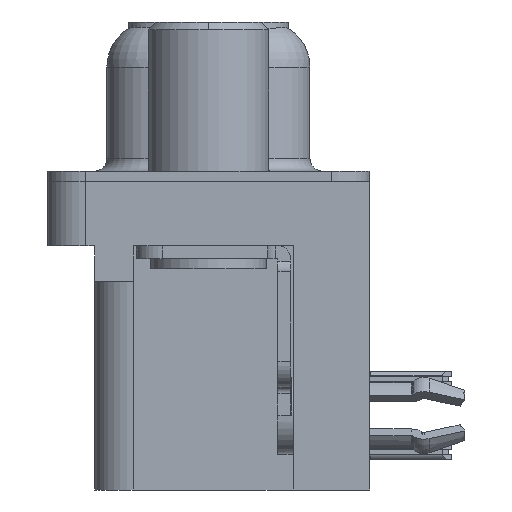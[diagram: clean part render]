
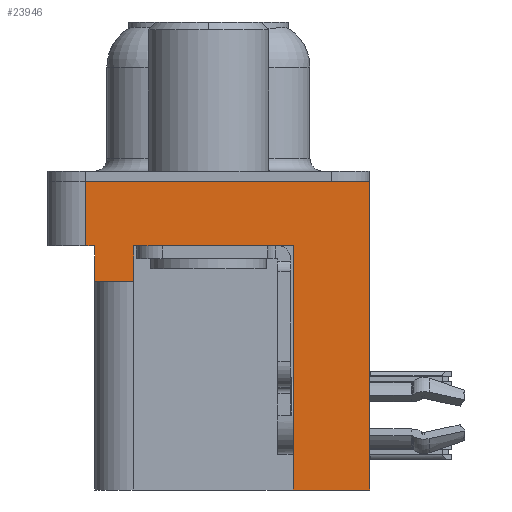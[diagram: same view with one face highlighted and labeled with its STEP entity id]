
A CAD part, left-side view. The second image highlights one B-rep face of the part: STEP entity #23946.
In plain terms, the highlighted planar face has unit normal (-1, 0, 0).
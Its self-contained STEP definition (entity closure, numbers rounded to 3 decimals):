
#235 = EDGE_CURVE ( 'NONE', #28378, #30935, #10967, .T. ) ;
#329 = LINE ( 'NONE', #23512, #26860 ) ;
#631 = AXIS2_PLACEMENT_3D ( 'NONE', #4601, #31173, #10521 ) ;
#839 = CARTESIAN_POINT ( 'NONE',  ( -2.91, 4.425, -3.9 ) ) ;
#1106 = DIRECTION ( 'NONE',  ( 0., 0., 1. ) ) ;
#1242 = LINE ( 'NONE', #29125, #35146 ) ;
#2614 = EDGE_CURVE ( 'NONE', #37680, #4108, #28813, .T. ) ;
#2791 = DIRECTION ( 'NONE',  ( 0., 1., 0. ) ) ;
#3628 = DIRECTION ( 'NONE',  ( 0., 0., 1. ) ) ;
#3944 = CARTESIAN_POINT ( 'NONE',  ( -2.91, 4.775, -2.5 ) ) ;
#4018 = VERTEX_POINT ( 'NONE', #26479 ) ;
#4051 = VECTOR ( 'NONE', #36265, 1000. ) ;
#4108 = VERTEX_POINT ( 'NONE', #20231 ) ;
#4146 = DIRECTION ( 'NONE',  ( 0., -1., 0. ) ) ;
#4537 = LINE ( 'NONE', #3944, #11026 ) ;
#4601 = CARTESIAN_POINT ( 'NONE',  ( -2.91, -6.275, -2.5 ) ) ;
#5103 = DIRECTION ( 'NONE',  ( 0., -1., 0. ) ) ;
#5271 = VECTOR ( 'NONE', #1106, 1000. ) ;
#5476 = CARTESIAN_POINT ( 'NONE',  ( -2.91, -3.295, -2.5 ) ) ;
#5695 = DIRECTION ( 'NONE',  ( 0., 0., 1. ) ) ;
#6063 = EDGE_CURVE ( 'NONE', #37680, #15336, #1242, .T. ) ;
#7387 = CARTESIAN_POINT ( 'NONE',  ( -2.91, 2.895, -2.5 ) ) ;
#7541 = LINE ( 'NONE', #839, #5271 ) ;
#7981 = ORIENTED_EDGE ( 'NONE', *, *, #6063, .F. ) ;
#8067 = CARTESIAN_POINT ( 'NONE',  ( -2.91, -6.275, -2.5 ) ) ;
#9348 = ORIENTED_EDGE ( 'NONE', *, *, #35114, .T. ) ;
#9843 = CARTESIAN_POINT ( 'NONE',  ( -2.91, -6.275, 0. ) ) ;
#10073 = CARTESIAN_POINT ( 'NONE',  ( -2.91, -6.275, -2.5 ) ) ;
#10372 = CARTESIAN_POINT ( 'NONE',  ( -2.91, 4.425, -2.5 ) ) ;
#10381 = PLANE ( 'NONE',  #631 ) ;
#10521 = DIRECTION ( 'NONE',  ( 0., 0., 1. ) ) ;
#10967 = LINE ( 'NONE', #24755, #36965 ) ;
#11026 = VECTOR ( 'NONE', #31152, 1000. ) ;
#11828 = DIRECTION ( 'NONE',  ( 0., 0., 1. ) ) ;
#12679 = ORIENTED_EDGE ( 'NONE', *, *, #37222, .F. ) ;
#13060 = VECTOR ( 'NONE', #11828, 1000. ) ;
#14082 = VECTOR ( 'NONE', #5103, 1000. ) ;
#14663 = CARTESIAN_POINT ( 'NONE',  ( -2.91, -6.275, -2.5 ) ) ;
#15336 = VERTEX_POINT ( 'NONE', #25518 ) ;
#17587 = VECTOR ( 'NONE', #4146, 1000. ) ;
#18052 = VERTEX_POINT ( 'NONE', #5476 ) ;
#18186 = VERTEX_POINT ( 'NONE', #20657 ) ;
#18630 = VERTEX_POINT ( 'NONE', #10372 ) ;
#18735 = CARTESIAN_POINT ( 'NONE',  ( -2.91, 2.895, -3.9 ) ) ;
#19504 = CARTESIAN_POINT ( 'NONE',  ( -2.91, 4.775, -2.5 ) ) ;
#19560 = ORIENTED_EDGE ( 'NONE', *, *, #27794, .F. ) ;
#20231 = CARTESIAN_POINT ( 'NONE',  ( -2.91, -6.275, 0. ) ) ;
#20316 = LINE ( 'NONE', #30776, #30576 ) ;
#20657 = CARTESIAN_POINT ( 'NONE',  ( -2.91, 4.775, 0. ) ) ;
#21347 = LINE ( 'NONE', #9843, #17587 ) ;
#21749 = CARTESIAN_POINT ( 'NONE',  ( -2.91, -6.275, -12. ) ) ;
#23512 = CARTESIAN_POINT ( 'NONE',  ( -2.91, -3.295, -12. ) ) ;
#23946 = ADVANCED_FACE ( 'NONE', ( #31598 ), #10381, .T. ) ;
#24593 = EDGE_CURVE ( 'NONE', #18186, #4108, #21347, .T. ) ;
#24753 = ORIENTED_EDGE ( 'NONE', *, *, #34754, .F. ) ;
#24755 = CARTESIAN_POINT ( 'NONE',  ( -2.91, 2.895, -3.9 ) ) ;
#25518 = CARTESIAN_POINT ( 'NONE',  ( -2.91, -3.295, -12. ) ) ;
#25639 = ORIENTED_EDGE ( 'NONE', *, *, #32097, .T. ) ;
#26312 = ORIENTED_EDGE ( 'NONE', *, *, #235, .T. ) ;
#26479 = CARTESIAN_POINT ( 'NONE',  ( -2.91, 4.425, -3.9 ) ) ;
#26794 = ORIENTED_EDGE ( 'NONE', *, *, #24593, .F. ) ;
#26860 = VECTOR ( 'NONE', #5695, 1000. ) ;
#27794 = EDGE_CURVE ( 'NONE', #28378, #4018, #20316, .T. ) ;
#28378 = VERTEX_POINT ( 'NONE', #18735 ) ;
#28499 = ORIENTED_EDGE ( 'NONE', *, *, #28740, .F. ) ;
#28740 = EDGE_CURVE ( 'NONE', #15336, #18052, #329, .T. ) ;
#28813 = LINE ( 'NONE', #14663, #13060 ) ;
#29075 = LINE ( 'NONE', #10073, #4051 ) ;
#29125 = CARTESIAN_POINT ( 'NONE',  ( -2.91, -3.295, -12. ) ) ;
#29463 = EDGE_LOOP ( 'NONE', ( #26794, #24753, #9348, #12679, #19560, #26312, #25639, #28499, #7981, #30219 ) ) ;
#30219 = ORIENTED_EDGE ( 'NONE', *, *, #2614, .T. ) ;
#30576 = VECTOR ( 'NONE', #30635, 1000. ) ;
#30635 = DIRECTION ( 'NONE',  ( 0., 1., 0. ) ) ;
#30776 = CARTESIAN_POINT ( 'NONE',  ( -2.91, 4.425, -3.9 ) ) ;
#30935 = VERTEX_POINT ( 'NONE', #7387 ) ;
#31152 = DIRECTION ( 'NONE',  ( 0., 0., 1. ) ) ;
#31173 = DIRECTION ( 'NONE',  ( -1., 0., 0. ) ) ;
#31598 = FACE_OUTER_BOUND ( 'NONE', #29463, .T. ) ;
#31926 = VERTEX_POINT ( 'NONE', #19504 ) ;
#32097 = EDGE_CURVE ( 'NONE', #30935, #18052, #32665, .T. ) ;
#32665 = LINE ( 'NONE', #8067, #14082 ) ;
#34754 = EDGE_CURVE ( 'NONE', #31926, #18186, #4537, .T. ) ;
#35114 = EDGE_CURVE ( 'NONE', #31926, #18630, #29075, .T. ) ;
#35146 = VECTOR ( 'NONE', #2791, 1000. ) ;
#36265 = DIRECTION ( 'NONE',  ( 0., -1., 0. ) ) ;
#36965 = VECTOR ( 'NONE', #3628, 1000. ) ;
#37222 = EDGE_CURVE ( 'NONE', #4018, #18630, #7541, .T. ) ;
#37680 = VERTEX_POINT ( 'NONE', #21749 ) ;
